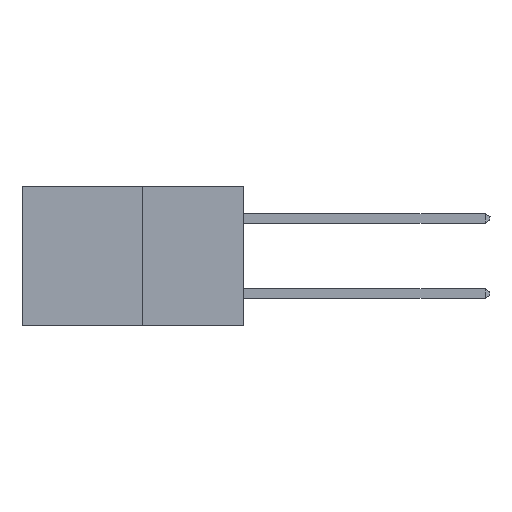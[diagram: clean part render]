
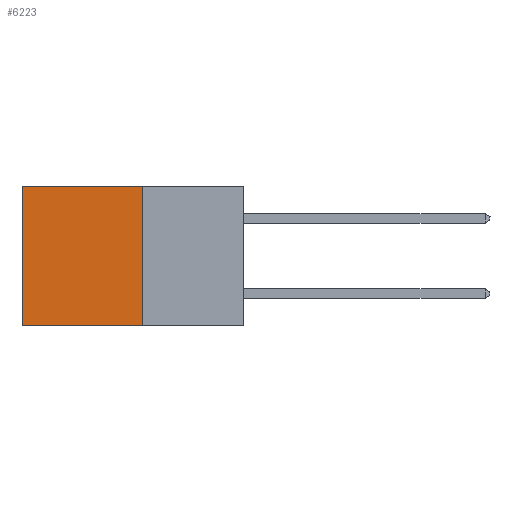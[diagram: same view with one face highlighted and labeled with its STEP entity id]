
A CAD part, left-side view. The second image highlights one B-rep face of the part: STEP entity #6223.
In plain terms, the highlighted planar face has unit normal (-1, 0, 0).
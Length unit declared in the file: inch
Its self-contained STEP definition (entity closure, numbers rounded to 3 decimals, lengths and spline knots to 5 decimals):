
#368 = CARTESIAN_POINT ( 'NONE',  ( 0.277, 0.27, -0.37 ) ) ;
#415 = ORIENTED_EDGE ( 'NONE', *, *, #9396, .T. ) ;
#936 = ORIENTED_EDGE ( 'NONE', *, *, #1856, .F. ) ;
#1023 = CARTESIAN_POINT ( 'NONE',  ( 0.277, 0.27, -0.37 ) ) ;
#1149 = VECTOR ( 'NONE', #5748, 39.37008 ) ;
#1406 = LINE ( 'NONE', #4409, #7026 ) ;
#1569 = DIRECTION ( 'NONE',  ( 0., 0., -1. ) ) ;
#1772 = FACE_OUTER_BOUND ( 'NONE', #8370, .T. ) ;
#1856 = EDGE_CURVE ( 'NONE', #2770, #9291, #1406, .T. ) ;
#1913 = VECTOR ( 'NONE', #1569, 39.37008 ) ;
#2120 = CARTESIAN_POINT ( 'NONE',  ( 0.277, 0.27, 0. ) ) ;
#2144 = VERTEX_POINT ( 'NONE', #4651 ) ;
#2312 = CARTESIAN_POINT ( 'NONE',  ( 0.277, 0.59, -0.37 ) ) ;
#2680 = EDGE_CURVE ( 'NONE', #9457, #2770, #5568, .T. ) ;
#2770 = VERTEX_POINT ( 'NONE', #1023 ) ;
#3286 = CARTESIAN_POINT ( 'NONE',  ( 0.277, 0.27, -0.37 ) ) ;
#4192 = DIRECTION ( 'NONE',  ( 0., 0., -1. ) ) ;
#4312 = LINE ( 'NONE', #2312, #5777 ) ;
#4409 = CARTESIAN_POINT ( 'NONE',  ( 0.277, 0.27, -0.37 ) ) ;
#4505 = DIRECTION ( 'NONE',  ( 0., 0., -1. ) ) ;
#4651 = CARTESIAN_POINT ( 'NONE',  ( 0.277, 0.59, 0. ) ) ;
#4921 = DIRECTION ( 'NONE',  ( 0., 1., 0. ) ) ;
#5241 = ORIENTED_EDGE ( 'NONE', *, *, #2680, .F. ) ;
#5568 = LINE ( 'NONE', #3286, #1913 ) ;
#5748 = DIRECTION ( 'NONE',  ( 0., 1., 0. ) ) ;
#5777 = VECTOR ( 'NONE', #4505, 39.37008 ) ;
#6104 = AXIS2_PLACEMENT_3D ( 'NONE', #368, #8471, #4192 ) ;
#6223 = ADVANCED_FACE ( 'NONE', ( #1772 ), #7064, .F. ) ;
#6465 = EDGE_CURVE ( 'NONE', #9457, #2144, #8878, .T. ) ;
#7026 = VECTOR ( 'NONE', #4921, 39.37008 ) ;
#7064 = PLANE ( 'NONE',  #6104 ) ;
#7423 = CARTESIAN_POINT ( 'NONE',  ( 0.277, 0.27, 0. ) ) ;
#8370 = EDGE_LOOP ( 'NONE', ( #415, #936, #5241, #8593 ) ) ;
#8471 = DIRECTION ( 'NONE',  ( 1., 0., 0. ) ) ;
#8593 = ORIENTED_EDGE ( 'NONE', *, *, #6465, .T. ) ;
#8655 = CARTESIAN_POINT ( 'NONE',  ( 0.277, 0.59, -0.37 ) ) ;
#8878 = LINE ( 'NONE', #2120, #1149 ) ;
#9291 = VERTEX_POINT ( 'NONE', #8655 ) ;
#9396 = EDGE_CURVE ( 'NONE', #2144, #9291, #4312, .T. ) ;
#9457 = VERTEX_POINT ( 'NONE', #7423 ) ;
